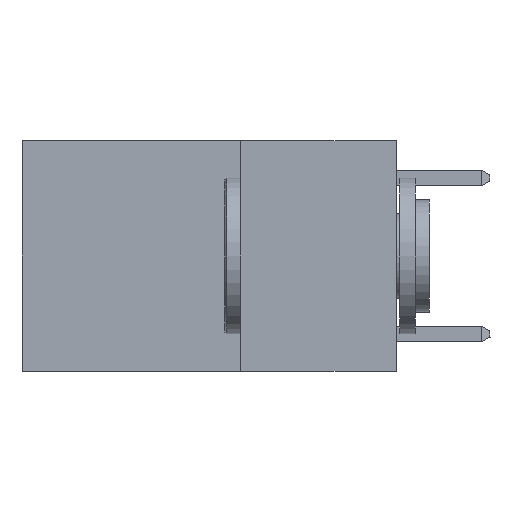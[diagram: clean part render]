
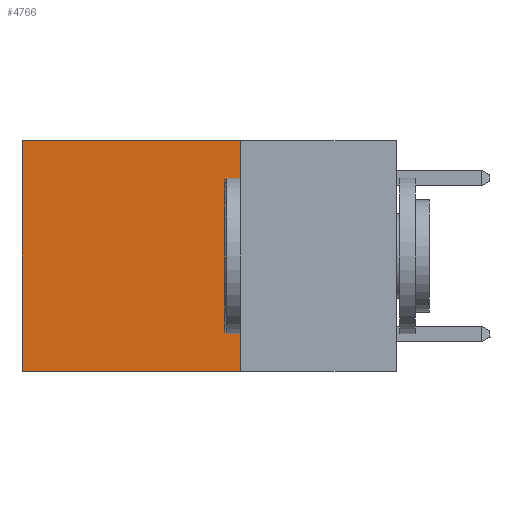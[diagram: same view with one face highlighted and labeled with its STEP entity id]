
A CAD part, left-side view. The second image highlights one B-rep face of the part: STEP entity #4766.
In plain terms, the highlighted planar face has unit normal (-1, 0, 0).
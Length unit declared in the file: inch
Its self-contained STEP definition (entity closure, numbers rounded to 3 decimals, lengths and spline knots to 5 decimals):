
#147 = VERTEX_POINT ( 'NONE', #944 ) ;
#285 = LINE ( 'NONE', #1673, #6814 ) ;
#382 = CARTESIAN_POINT ( 'NONE',  ( 0.2625, 0.25, 0. ) ) ;
#519 = ORIENTED_EDGE ( 'NONE', *, *, #9068, .T. ) ;
#663 = LINE ( 'NONE', #7797, #5014 ) ;
#861 = DIRECTION ( 'NONE',  ( 1., 0., 0. ) ) ;
#944 = CARTESIAN_POINT ( 'NONE',  ( 0.2625, 0.25, -0.37 ) ) ;
#1295 = DIRECTION ( 'NONE',  ( 0., 1., 0. ) ) ;
#1671 = DIRECTION ( 'NONE',  ( 0., 1., 0. ) ) ;
#1673 = CARTESIAN_POINT ( 'NONE',  ( 0.2625, 0.25, 0. ) ) ;
#1962 = VERTEX_POINT ( 'NONE', #7457 ) ;
#2359 = VECTOR ( 'NONE', #9237, 39.37008 ) ;
#2668 = VECTOR ( 'NONE', #1671, 39.37008 ) ;
#2909 = CARTESIAN_POINT ( 'NONE',  ( 0.2625, 0.6, 0. ) ) ;
#3087 = CARTESIAN_POINT ( 'NONE',  ( 0.2625, 0.25, -0.37 ) ) ;
#3270 = ORIENTED_EDGE ( 'NONE', *, *, #8770, .F. ) ;
#3382 = ORIENTED_EDGE ( 'NONE', *, *, #4565, .T. ) ;
#3626 = LINE ( 'NONE', #2909, #2359 ) ;
#3853 = CARTESIAN_POINT ( 'NONE',  ( 0.2625, 0.25, 0. ) ) ;
#4367 = ORIENTED_EDGE ( 'NONE', *, *, #5970, .F. ) ;
#4495 = VERTEX_POINT ( 'NONE', #8285 ) ;
#4540 = LINE ( 'NONE', #3087, #2668 ) ;
#4565 = EDGE_CURVE ( 'NONE', #1962, #4495, #3626, .T. ) ;
#4766 = ADVANCED_FACE ( 'NONE', ( #7482 ), #8091, .F. ) ;
#5014 = VECTOR ( 'NONE', #1295, 39.37008 ) ;
#5726 = VERTEX_POINT ( 'NONE', #382 ) ;
#5970 = EDGE_CURVE ( 'NONE', #147, #4495, #4540, .T. ) ;
#6575 = AXIS2_PLACEMENT_3D ( 'NONE', #3853, #861, #8183 ) ;
#6814 = VECTOR ( 'NONE', #8143, 39.37008 ) ;
#7457 = CARTESIAN_POINT ( 'NONE',  ( 0.2625, 0.6, 0. ) ) ;
#7482 = FACE_OUTER_BOUND ( 'NONE', #9164, .T. ) ;
#7797 = CARTESIAN_POINT ( 'NONE',  ( 0.2625, 0.25, 0. ) ) ;
#8091 = PLANE ( 'NONE',  #6575 ) ;
#8143 = DIRECTION ( 'NONE',  ( 0., 0., -1. ) ) ;
#8183 = DIRECTION ( 'NONE',  ( 0., 0., -1. ) ) ;
#8285 = CARTESIAN_POINT ( 'NONE',  ( 0.2625, 0.6, -0.37 ) ) ;
#8770 = EDGE_CURVE ( 'NONE', #5726, #147, #285, .T. ) ;
#9068 = EDGE_CURVE ( 'NONE', #5726, #1962, #663, .T. ) ;
#9164 = EDGE_LOOP ( 'NONE', ( #3382, #4367, #3270, #519 ) ) ;
#9237 = DIRECTION ( 'NONE',  ( 0., 0., -1. ) ) ;
